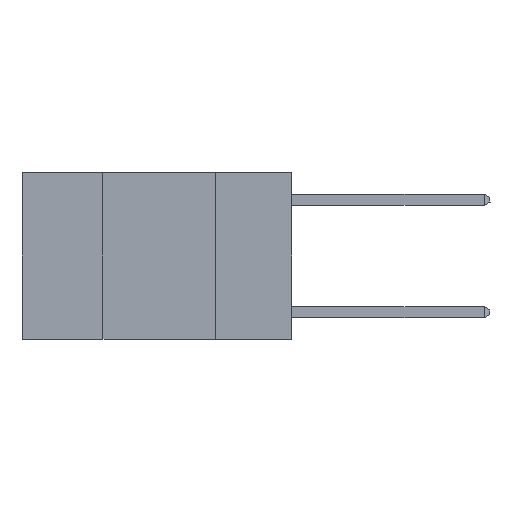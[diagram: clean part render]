
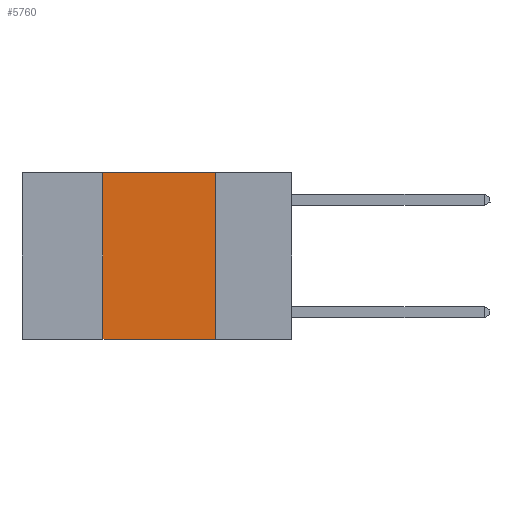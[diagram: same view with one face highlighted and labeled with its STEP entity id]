
A CAD part, left-side view. The second image highlights one B-rep face of the part: STEP entity #5760.
In plain terms, the highlighted planar face has unit normal (-1, 0, 0).
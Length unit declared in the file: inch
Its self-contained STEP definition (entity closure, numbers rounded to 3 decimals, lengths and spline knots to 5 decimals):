
#245 = ORIENTED_EDGE ( 'NONE', *, *, #3016, .F. ) ;
#413 = DIRECTION ( 'NONE',  ( 0., -1., 0. ) ) ;
#578 = VERTEX_POINT ( 'NONE', #2374 ) ;
#1002 = VERTEX_POINT ( 'NONE', #7165 ) ;
#1837 = LINE ( 'NONE', #4356, #4939 ) ;
#2125 = VECTOR ( 'NONE', #7275, 39.37008 ) ;
#2332 = ORIENTED_EDGE ( 'NONE', *, *, #6599, .F. ) ;
#2374 = CARTESIAN_POINT ( 'NONE',  ( 0., 0.17, -0.37 ) ) ;
#3016 = EDGE_CURVE ( 'NONE', #1002, #5251, #3327, .T. ) ;
#3327 = LINE ( 'NONE', #16924, #14530 ) ;
#4241 = CARTESIAN_POINT ( 'NONE',  ( 0., 0.6, 0. ) ) ;
#4356 = CARTESIAN_POINT ( 'NONE',  ( 0., 0.42, 0. ) ) ;
#4939 = VECTOR ( 'NONE', #5717, 39.37008 ) ;
#5251 = VERTEX_POINT ( 'NONE', #15380 ) ;
#5590 = DIRECTION ( 'NONE',  ( 1., 0., 0. ) ) ;
#5717 = DIRECTION ( 'NONE',  ( 0., 0., 1. ) ) ;
#5760 = ADVANCED_FACE ( 'NONE', ( #15782 ), #13696, .F. ) ;
#6599 = EDGE_CURVE ( 'NONE', #15930, #1002, #1837, .T. ) ;
#7165 = CARTESIAN_POINT ( 'NONE',  ( 0., 0.42, 0. ) ) ;
#7275 = DIRECTION ( 'NONE',  ( 0., 0., -1. ) ) ;
#8735 = DIRECTION ( 'NONE',  ( 0., -1., 0. ) ) ;
#9147 = CARTESIAN_POINT ( 'NONE',  ( 0., 0.42, -0.37 ) ) ;
#9602 = LINE ( 'NONE', #16799, #2125 ) ;
#11539 = VECTOR ( 'NONE', #413, 39.37008 ) ;
#11717 = ORIENTED_EDGE ( 'NONE', *, *, #13139, .T. ) ;
#12243 = AXIS2_PLACEMENT_3D ( 'NONE', #4241, #5590, #15077 ) ;
#12360 = EDGE_LOOP ( 'NONE', ( #17077, #245, #2332, #11717 ) ) ;
#12562 = EDGE_CURVE ( 'NONE', #5251, #578, #9602, .T. ) ;
#13139 = EDGE_CURVE ( 'NONE', #15930, #578, #15202, .T. ) ;
#13696 = PLANE ( 'NONE',  #12243 ) ;
#14530 = VECTOR ( 'NONE', #8735, 39.37008 ) ;
#15040 = CARTESIAN_POINT ( 'NONE',  ( 0., 0.6, -0.37 ) ) ;
#15077 = DIRECTION ( 'NONE',  ( 0., 0., -1. ) ) ;
#15202 = LINE ( 'NONE', #15040, #11539 ) ;
#15380 = CARTESIAN_POINT ( 'NONE',  ( 0., 0.17, 0. ) ) ;
#15782 = FACE_OUTER_BOUND ( 'NONE', #12360, .T. ) ;
#15930 = VERTEX_POINT ( 'NONE', #9147 ) ;
#16799 = CARTESIAN_POINT ( 'NONE',  ( 0., 0.17, 0. ) ) ;
#16924 = CARTESIAN_POINT ( 'NONE',  ( 0., 0.6, 0. ) ) ;
#17077 = ORIENTED_EDGE ( 'NONE', *, *, #12562, .F. ) ;
